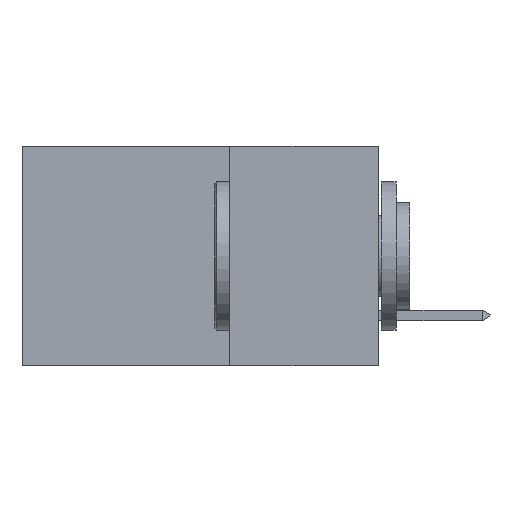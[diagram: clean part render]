
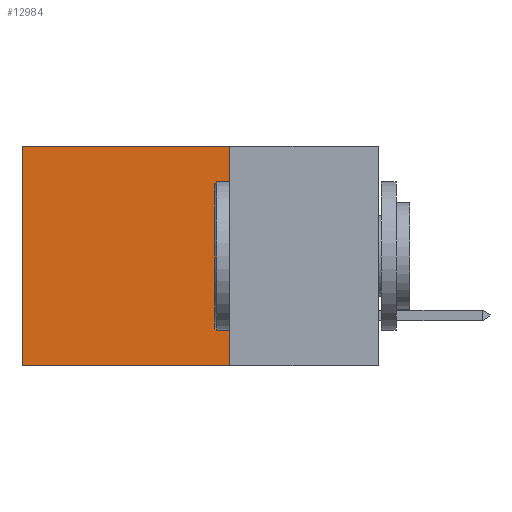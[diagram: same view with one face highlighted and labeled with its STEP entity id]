
A CAD part, left-side view. The second image highlights one B-rep face of the part: STEP entity #12984.
In plain terms, the highlighted planar face has unit normal (-1, 0, 0).
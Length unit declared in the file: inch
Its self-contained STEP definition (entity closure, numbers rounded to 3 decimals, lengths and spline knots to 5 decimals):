
#155 = DIRECTION ( 'NONE',  ( 0., 1., 0. ) ) ;
#669 = ORIENTED_EDGE ( 'NONE', *, *, #19682, .F. ) ;
#975 = VERTEX_POINT ( 'NONE', #24459 ) ;
#1043 = CARTESIAN_POINT ( 'NONE',  ( 0.2615, 0.25, -0.37 ) ) ;
#1273 = EDGE_CURVE ( 'NONE', #13230, #23334, #6555, .T. ) ;
#1990 = EDGE_CURVE ( 'NONE', #5594, #975, #6493, .T. ) ;
#2150 = DIRECTION ( 'NONE',  ( 0., 1., 0. ) ) ;
#2818 = EDGE_CURVE ( 'NONE', #13230, #5594, #6186, .T. ) ;
#5594 = VERTEX_POINT ( 'NONE', #23033 ) ;
#5680 = CARTESIAN_POINT ( 'NONE',  ( 0.2615, 0.25, -0.37 ) ) ;
#6186 = LINE ( 'NONE', #8339, #8670 ) ;
#6493 = LINE ( 'NONE', #12055, #20242 ) ;
#6555 = LINE ( 'NONE', #7861, #19367 ) ;
#7386 = CARTESIAN_POINT ( 'NONE',  ( 0.2615, 0.25, -0.37 ) ) ;
#7861 = CARTESIAN_POINT ( 'NONE',  ( 0.2615, 0.25, -0.37 ) ) ;
#8339 = CARTESIAN_POINT ( 'NONE',  ( 0.2615, 0.25, 0. ) ) ;
#8500 = DIRECTION ( 'NONE',  ( 1., 0., 0. ) ) ;
#8585 = ORIENTED_EDGE ( 'NONE', *, *, #2818, .T. ) ;
#8670 = VECTOR ( 'NONE', #2150, 39.37008 ) ;
#10521 = PLANE ( 'NONE',  #16910 ) ;
#12055 = CARTESIAN_POINT ( 'NONE',  ( 0.2615, 0.6, -0.37 ) ) ;
#12984 = ADVANCED_FACE ( 'NONE', ( #20384 ), #10521, .F. ) ;
#13230 = VERTEX_POINT ( 'NONE', #21230 ) ;
#14070 = DIRECTION ( 'NONE',  ( 0., 0., -1. ) ) ;
#15859 = DIRECTION ( 'NONE',  ( 0., 0., -1. ) ) ;
#16910 = AXIS2_PLACEMENT_3D ( 'NONE', #1043, #8500, #14070 ) ;
#17362 = LINE ( 'NONE', #7386, #21503 ) ;
#19367 = VECTOR ( 'NONE', #23644, 39.37008 ) ;
#19682 = EDGE_CURVE ( 'NONE', #23334, #975, #17362, .T. ) ;
#20118 = ORIENTED_EDGE ( 'NONE', *, *, #1990, .T. ) ;
#20242 = VECTOR ( 'NONE', #15859, 39.37008 ) ;
#20384 = FACE_OUTER_BOUND ( 'NONE', #24578, .T. ) ;
#21230 = CARTESIAN_POINT ( 'NONE',  ( 0.2615, 0.25, 0. ) ) ;
#21503 = VECTOR ( 'NONE', #155, 39.37008 ) ;
#21579 = ORIENTED_EDGE ( 'NONE', *, *, #1273, .F. ) ;
#23033 = CARTESIAN_POINT ( 'NONE',  ( 0.2615, 0.6, 0. ) ) ;
#23334 = VERTEX_POINT ( 'NONE', #5680 ) ;
#23644 = DIRECTION ( 'NONE',  ( 0., 0., -1. ) ) ;
#24459 = CARTESIAN_POINT ( 'NONE',  ( 0.2615, 0.6, -0.37 ) ) ;
#24578 = EDGE_LOOP ( 'NONE', ( #20118, #669, #21579, #8585 ) ) ;
